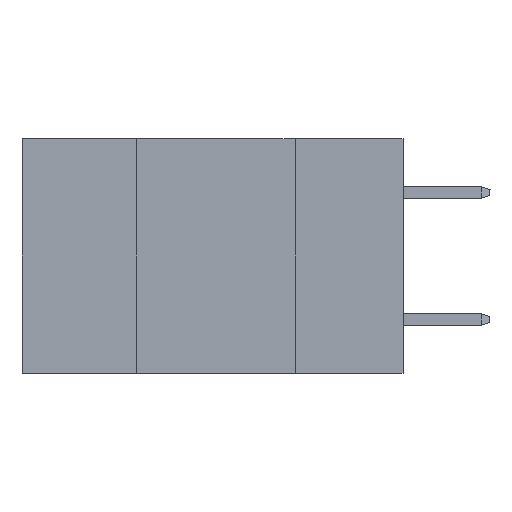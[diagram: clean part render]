
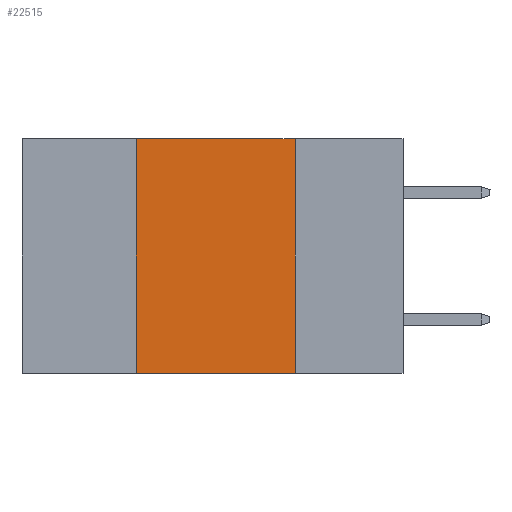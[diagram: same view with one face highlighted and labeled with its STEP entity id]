
A CAD part, left-side view. The second image highlights one B-rep face of the part: STEP entity #22515.
In plain terms, the highlighted planar face has unit normal (-1, 0, 0).
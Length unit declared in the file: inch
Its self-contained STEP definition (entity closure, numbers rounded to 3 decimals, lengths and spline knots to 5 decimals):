
#1349 = CARTESIAN_POINT ( 'NONE',  ( 0., 0.6, 0. ) ) ;
#3057 = FACE_OUTER_BOUND ( 'NONE', #25971, .T. ) ;
#3485 = AXIS2_PLACEMENT_3D ( 'NONE', #21020, #19145, #15438 ) ;
#3780 = VERTEX_POINT ( 'NONE', #7812 ) ;
#3890 = DIRECTION ( 'NONE',  ( 0., -1., 0. ) ) ;
#5685 = VERTEX_POINT ( 'NONE', #22871 ) ;
#5785 = ORIENTED_EDGE ( 'NONE', *, *, #15839, .F. ) ;
#6443 = VECTOR ( 'NONE', #3890, 39.37008 ) ;
#7503 = VECTOR ( 'NONE', #25735, 39.37008 ) ;
#7812 = CARTESIAN_POINT ( 'NONE',  ( 0., 0.17, 0. ) ) ;
#8467 = EDGE_CURVE ( 'NONE', #5685, #3780, #11267, .T. ) ;
#11267 = LINE ( 'NONE', #1349, #13977 ) ;
#11782 = LINE ( 'NONE', #22214, #7503 ) ;
#12899 = ORIENTED_EDGE ( 'NONE', *, *, #8467, .F. ) ;
#13162 = CARTESIAN_POINT ( 'NONE',  ( 0., 0.17, -0.37 ) ) ;
#13224 = DIRECTION ( 'NONE',  ( 0., -1., 0. ) ) ;
#13895 = CARTESIAN_POINT ( 'NONE',  ( 0., 0.6, -0.37 ) ) ;
#13977 = VECTOR ( 'NONE', #13224, 39.37008 ) ;
#14597 = VERTEX_POINT ( 'NONE', #13162 ) ;
#14703 = LINE ( 'NONE', #19057, #21833 ) ;
#14996 = EDGE_CURVE ( 'NONE', #3780, #14597, #14703, .T. ) ;
#15438 = DIRECTION ( 'NONE',  ( 0., 0., -1. ) ) ;
#15456 = VERTEX_POINT ( 'NONE', #19025 ) ;
#15839 = EDGE_CURVE ( 'NONE', #15456, #5685, #11782, .T. ) ;
#19025 = CARTESIAN_POINT ( 'NONE',  ( 0., 0.42, -0.37 ) ) ;
#19057 = CARTESIAN_POINT ( 'NONE',  ( 0., 0.17, 0. ) ) ;
#19145 = DIRECTION ( 'NONE',  ( 1., 0., 0. ) ) ;
#19750 = ORIENTED_EDGE ( 'NONE', *, *, #24282, .T. ) ;
#21020 = CARTESIAN_POINT ( 'NONE',  ( 0., 0.6, 0. ) ) ;
#21291 = PLANE ( 'NONE',  #3485 ) ;
#21833 = VECTOR ( 'NONE', #22785, 39.37008 ) ;
#22214 = CARTESIAN_POINT ( 'NONE',  ( 0., 0.42, 0. ) ) ;
#22351 = LINE ( 'NONE', #13895, #6443 ) ;
#22515 = ADVANCED_FACE ( 'NONE', ( #3057 ), #21291, .F. ) ;
#22785 = DIRECTION ( 'NONE',  ( 0., 0., -1. ) ) ;
#22871 = CARTESIAN_POINT ( 'NONE',  ( 0., 0.42, 0. ) ) ;
#24282 = EDGE_CURVE ( 'NONE', #15456, #14597, #22351, .T. ) ;
#25735 = DIRECTION ( 'NONE',  ( 0., 0., 1. ) ) ;
#25942 = ORIENTED_EDGE ( 'NONE', *, *, #14996, .F. ) ;
#25971 = EDGE_LOOP ( 'NONE', ( #25942, #12899, #5785, #19750 ) ) ;
